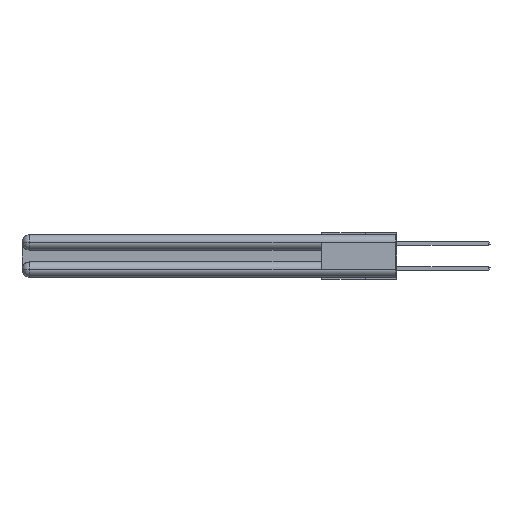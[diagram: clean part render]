
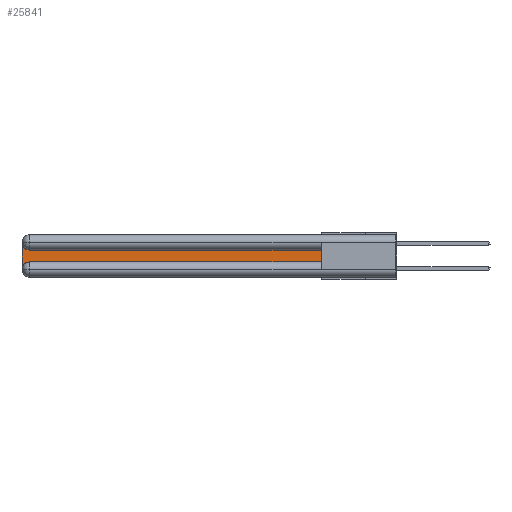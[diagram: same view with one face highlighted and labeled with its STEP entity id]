
A CAD part, left-side view. The second image highlights one B-rep face of the part: STEP entity #25841.
In plain terms, the highlighted planar face has unit normal (-1, 0, 0).
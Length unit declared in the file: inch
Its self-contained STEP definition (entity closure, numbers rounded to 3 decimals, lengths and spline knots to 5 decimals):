
#263 = LINE ( 'NONE', #12067, #20195 ) ;
#2405 = AXIS2_PLACEMENT_3D ( 'NONE', #15707, #13207, #7947 ) ;
#2418 = ORIENTED_EDGE ( 'NONE', *, *, #29624, .T. ) ;
#2683 = VECTOR ( 'NONE', #14473, 39.37008 ) ;
#3090 = LINE ( 'NONE', #9446, #2683 ) ;
#3648 = VERTEX_POINT ( 'NONE', #7309 ) ;
#3772 = EDGE_CURVE ( 'NONE', #31656, #27374, #28864, .T. ) ;
#4026 = EDGE_CURVE ( 'NONE', #3648, #30328, #263, .T. ) ;
#4249 = DIRECTION ( 'NONE',  ( 0., 0., -1. ) ) ;
#4802 = EDGE_CURVE ( 'NONE', #22686, #3648, #12334, .T. ) ;
#5767 = CARTESIAN_POINT ( 'NONE',  ( 0.075, 0.6, -0.2175 ) ) ;
#5888 = DIRECTION ( 'NONE',  ( 1., 0., 0. ) ) ;
#6073 = DIRECTION ( 'NONE',  ( 0., -1., 0. ) ) ;
#7309 = CARTESIAN_POINT ( 'NONE',  ( 0.075, 3., -0.0625 ) ) ;
#7947 = DIRECTION ( 'NONE',  ( 0., 0., -1. ) ) ;
#8102 = ORIENTED_EDGE ( 'NONE', *, *, #4802, .T. ) ;
#8475 = FACE_OUTER_BOUND ( 'NONE', #23627, .T. ) ;
#9446 = CARTESIAN_POINT ( 'NONE',  ( 0.075, 0.6, -0.1225 ) ) ;
#12067 = CARTESIAN_POINT ( 'NONE',  ( 0.075, 3., -0.2175 ) ) ;
#12334 = CIRCLE ( 'NONE', #32009, 0.06 ) ;
#12441 = ORIENTED_EDGE ( 'NONE', *, *, #3772, .T. ) ;
#12798 = CARTESIAN_POINT ( 'NONE',  ( 0.075, 2.94, -0.1225 ) ) ;
#13142 = DIRECTION ( 'NONE',  ( 0., 0., -1. ) ) ;
#13207 = DIRECTION ( 'NONE',  ( 1., 0., 0. ) ) ;
#14269 = EDGE_CURVE ( 'NONE', #27374, #22686, #3090, .T. ) ;
#14473 = DIRECTION ( 'NONE',  ( 0., 1., 0. ) ) ;
#14996 = ORIENTED_EDGE ( 'NONE', *, *, #14269, .T. ) ;
#15239 = VERTEX_POINT ( 'NONE', #27106 ) ;
#15707 = CARTESIAN_POINT ( 'NONE',  ( 0.075, 3., -0.1225 ) ) ;
#15955 = CARTESIAN_POINT ( 'NONE',  ( 0.075, 2.94, -0.0625 ) ) ;
#16043 = CIRCLE ( 'NONE', #28041, 0.06 ) ;
#16711 = DIRECTION ( 'NONE',  ( 1., 0., 0. ) ) ;
#20195 = VECTOR ( 'NONE', #27575, 39.37008 ) ;
#20993 = VECTOR ( 'NONE', #6073, 39.37008 ) ;
#21189 = ORIENTED_EDGE ( 'NONE', *, *, #25492, .T. ) ;
#21277 = CARTESIAN_POINT ( 'NONE',  ( 0.075, 2.94, -0.2775 ) ) ;
#22287 = CARTESIAN_POINT ( 'NONE',  ( 0.075, 0.6, -0.1225 ) ) ;
#22686 = VERTEX_POINT ( 'NONE', #12798 ) ;
#23341 = CARTESIAN_POINT ( 'NONE',  ( 0.075, 3., -0.2775 ) ) ;
#23402 = ORIENTED_EDGE ( 'NONE', *, *, #4026, .T. ) ;
#23627 = EDGE_LOOP ( 'NONE', ( #14996, #8102, #23402, #2418, #21189, #12441 ) ) ;
#25444 = PLANE ( 'NONE',  #2405 ) ;
#25492 = EDGE_CURVE ( 'NONE', #15239, #31656, #28492, .T. ) ;
#25743 = CARTESIAN_POINT ( 'NONE',  ( 0.075, 0.6, -0.2175 ) ) ;
#25841 = ADVANCED_FACE ( 'NONE', ( #8475 ), #25444, .F. ) ;
#27106 = CARTESIAN_POINT ( 'NONE',  ( 0.075, 2.94, -0.2175 ) ) ;
#27374 = VERTEX_POINT ( 'NONE', #22287 ) ;
#27575 = DIRECTION ( 'NONE',  ( 0., 0., -1. ) ) ;
#28041 = AXIS2_PLACEMENT_3D ( 'NONE', #21277, #16711, #4249 ) ;
#28059 = DIRECTION ( 'NONE',  ( 0., 0., 1. ) ) ;
#28492 = LINE ( 'NONE', #5767, #20993 ) ;
#28864 = LINE ( 'NONE', #25743, #29261 ) ;
#29261 = VECTOR ( 'NONE', #28059, 39.37008 ) ;
#29624 = EDGE_CURVE ( 'NONE', #30328, #15239, #16043, .T. ) ;
#30328 = VERTEX_POINT ( 'NONE', #23341 ) ;
#30832 = CARTESIAN_POINT ( 'NONE',  ( 0.075, 0.6, -0.2175 ) ) ;
#31656 = VERTEX_POINT ( 'NONE', #30832 ) ;
#32009 = AXIS2_PLACEMENT_3D ( 'NONE', #15955, #5888, #13142 ) ;
